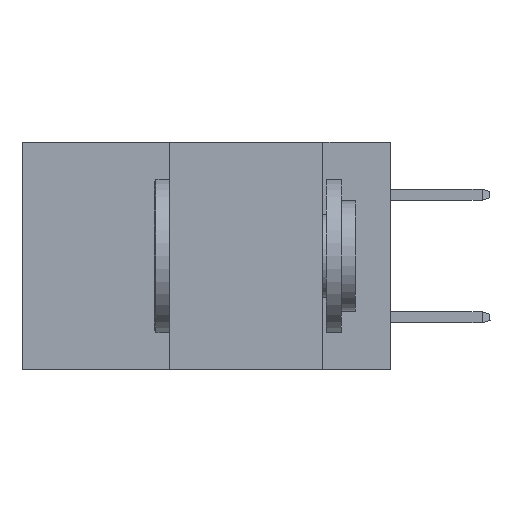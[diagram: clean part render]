
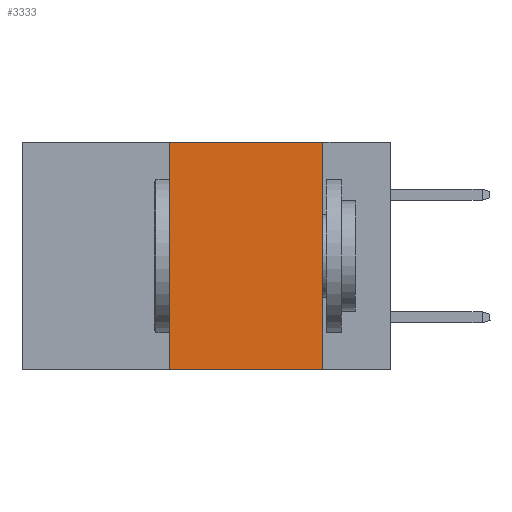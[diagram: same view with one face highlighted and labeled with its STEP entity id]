
A CAD part, left-side view. The second image highlights one B-rep face of the part: STEP entity #3333.
In plain terms, the highlighted planar face has unit normal (-1, 0, 0).
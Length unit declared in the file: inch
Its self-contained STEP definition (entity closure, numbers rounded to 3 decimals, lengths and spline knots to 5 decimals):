
#951 = VECTOR ( 'NONE', #20069, 39.37008 ) ;
#2015 = PLANE ( 'NONE',  #2239 ) ;
#2239 = AXIS2_PLACEMENT_3D ( 'NONE', #21246, #17394, #17591 ) ;
#2587 = LINE ( 'NONE', #16438, #15843 ) ;
#3069 = VERTEX_POINT ( 'NONE', #27279 ) ;
#3185 = ORIENTED_EDGE ( 'NONE', *, *, #5310, .F. ) ;
#3333 = ADVANCED_FACE ( 'NONE', ( #8300 ), #2015, .F. ) ;
#5310 = EDGE_CURVE ( 'NONE', #27406, #16116, #2587, .T. ) ;
#5554 = EDGE_LOOP ( 'NONE', ( #8722, #8723, #3185, #21867 ) ) ;
#7575 = DIRECTION ( 'NONE',  ( 0., 0., 1. ) ) ;
#7975 = CARTESIAN_POINT ( 'NONE',  ( 0., 0.11, -0.37 ) ) ;
#8300 = FACE_OUTER_BOUND ( 'NONE', #5554, .T. ) ;
#8722 = ORIENTED_EDGE ( 'NONE', *, *, #13938, .F. ) ;
#8723 = ORIENTED_EDGE ( 'NONE', *, *, #17536, .F. ) ;
#9702 = CARTESIAN_POINT ( 'NONE',  ( 0., 0.6, -0.37 ) ) ;
#13117 = CARTESIAN_POINT ( 'NONE',  ( 0., 0.11, 0. ) ) ;
#13938 = EDGE_CURVE ( 'NONE', #3069, #27873, #21793, .T. ) ;
#15062 = LINE ( 'NONE', #18367, #26159 ) ;
#15843 = VECTOR ( 'NONE', #7575, 39.37008 ) ;
#16116 = VERTEX_POINT ( 'NONE', #28615 ) ;
#16438 = CARTESIAN_POINT ( 'NONE',  ( 0., 0.36, 0. ) ) ;
#16614 = DIRECTION ( 'NONE',  ( 0., -1., 0. ) ) ;
#17394 = DIRECTION ( 'NONE',  ( 1., 0., 0. ) ) ;
#17536 = EDGE_CURVE ( 'NONE', #16116, #3069, #15062, .T. ) ;
#17591 = DIRECTION ( 'NONE',  ( 0., 0., -1. ) ) ;
#18367 = CARTESIAN_POINT ( 'NONE',  ( 0., 0.6, 0. ) ) ;
#18725 = LINE ( 'NONE', #9702, #24233 ) ;
#20069 = DIRECTION ( 'NONE',  ( 0., 0., -1. ) ) ;
#21246 = CARTESIAN_POINT ( 'NONE',  ( 0., 0.6, 0. ) ) ;
#21793 = LINE ( 'NONE', #13117, #951 ) ;
#21867 = ORIENTED_EDGE ( 'NONE', *, *, #27269, .T. ) ;
#22682 = DIRECTION ( 'NONE',  ( 0., -1., 0. ) ) ;
#24233 = VECTOR ( 'NONE', #16614, 39.37008 ) ;
#26159 = VECTOR ( 'NONE', #22682, 39.37008 ) ;
#27269 = EDGE_CURVE ( 'NONE', #27406, #27873, #18725, .T. ) ;
#27279 = CARTESIAN_POINT ( 'NONE',  ( 0., 0.11, 0. ) ) ;
#27406 = VERTEX_POINT ( 'NONE', #28321 ) ;
#27873 = VERTEX_POINT ( 'NONE', #7975 ) ;
#28321 = CARTESIAN_POINT ( 'NONE',  ( 0., 0.36, -0.37 ) ) ;
#28615 = CARTESIAN_POINT ( 'NONE',  ( 0., 0.36, 0. ) ) ;
